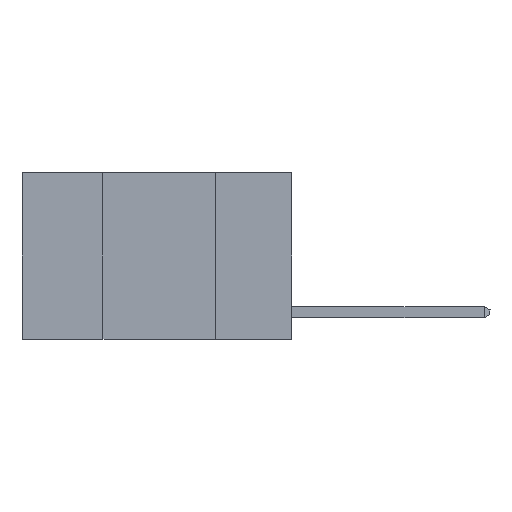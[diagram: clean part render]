
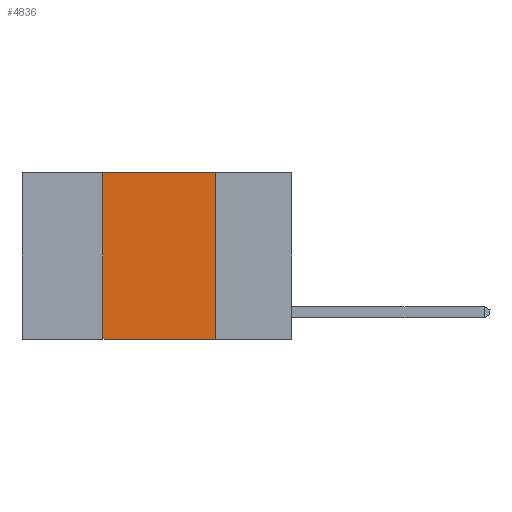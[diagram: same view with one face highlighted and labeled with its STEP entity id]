
A CAD part, left-side view. The second image highlights one B-rep face of the part: STEP entity #4836.
In plain terms, the highlighted planar face has unit normal (-1, 0, 0).
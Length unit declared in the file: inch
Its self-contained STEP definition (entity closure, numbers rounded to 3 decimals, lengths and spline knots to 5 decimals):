
#1216 = EDGE_CURVE ( 'NONE', #1989, #5242, #3481, .T. ) ;
#1450 = CARTESIAN_POINT ( 'NONE',  ( 0., 0.17, 0. ) ) ;
#1989 = VERTEX_POINT ( 'NONE', #2337 ) ;
#2011 = CARTESIAN_POINT ( 'NONE',  ( 0., 0.6, 0. ) ) ;
#2337 = CARTESIAN_POINT ( 'NONE',  ( 0., 0.17, 0. ) ) ;
#2789 = DIRECTION ( 'NONE',  ( 0., -1., 0. ) ) ;
#3004 = VERTEX_POINT ( 'NONE', #19988 ) ;
#3481 = LINE ( 'NONE', #1450, #10914 ) ;
#4357 = LINE ( 'NONE', #19625, #14597 ) ;
#4836 = ADVANCED_FACE ( 'NONE', ( #16332 ), #13829, .F. ) ;
#4911 = VECTOR ( 'NONE', #28527, 39.37008 ) ;
#5242 = VERTEX_POINT ( 'NONE', #9885 ) ;
#5445 = ORIENTED_EDGE ( 'NONE', *, *, #1216, .F. ) ;
#5996 = CARTESIAN_POINT ( 'NONE',  ( 0., 0.42, 0. ) ) ;
#6228 = AXIS2_PLACEMENT_3D ( 'NONE', #2011, #6374, #18690 ) ;
#6307 = LINE ( 'NONE', #5996, #30017 ) ;
#6374 = DIRECTION ( 'NONE',  ( 1., 0., 0. ) ) ;
#8326 = DIRECTION ( 'NONE',  ( 0., 0., 1. ) ) ;
#8459 = DIRECTION ( 'NONE',  ( 0., 0., -1. ) ) ;
#9885 = CARTESIAN_POINT ( 'NONE',  ( 0., 0.17, -0.37 ) ) ;
#10374 = ORIENTED_EDGE ( 'NONE', *, *, #18577, .F. ) ;
#10914 = VECTOR ( 'NONE', #8459, 39.37008 ) ;
#12074 = ORIENTED_EDGE ( 'NONE', *, *, #12414, .T. ) ;
#12414 = EDGE_CURVE ( 'NONE', #3004, #5242, #4357, .T. ) ;
#13829 = PLANE ( 'NONE',  #6228 ) ;
#14597 = VECTOR ( 'NONE', #2789, 39.37008 ) ;
#15651 = ORIENTED_EDGE ( 'NONE', *, *, #27091, .F. ) ;
#16332 = FACE_OUTER_BOUND ( 'NONE', #19912, .T. ) ;
#16658 = LINE ( 'NONE', #17273, #4911 ) ;
#17273 = CARTESIAN_POINT ( 'NONE',  ( 0., 0.6, 0. ) ) ;
#18577 = EDGE_CURVE ( 'NONE', #3004, #30645, #6307, .T. ) ;
#18690 = DIRECTION ( 'NONE',  ( 0., 0., -1. ) ) ;
#19625 = CARTESIAN_POINT ( 'NONE',  ( 0., 0.6, -0.37 ) ) ;
#19912 = EDGE_LOOP ( 'NONE', ( #5445, #15651, #10374, #12074 ) ) ;
#19988 = CARTESIAN_POINT ( 'NONE',  ( 0., 0.42, -0.37 ) ) ;
#27091 = EDGE_CURVE ( 'NONE', #30645, #1989, #16658, .T. ) ;
#28527 = DIRECTION ( 'NONE',  ( 0., -1., 0. ) ) ;
#29465 = CARTESIAN_POINT ( 'NONE',  ( 0., 0.42, 0. ) ) ;
#30017 = VECTOR ( 'NONE', #8326, 39.37008 ) ;
#30645 = VERTEX_POINT ( 'NONE', #29465 ) ;
